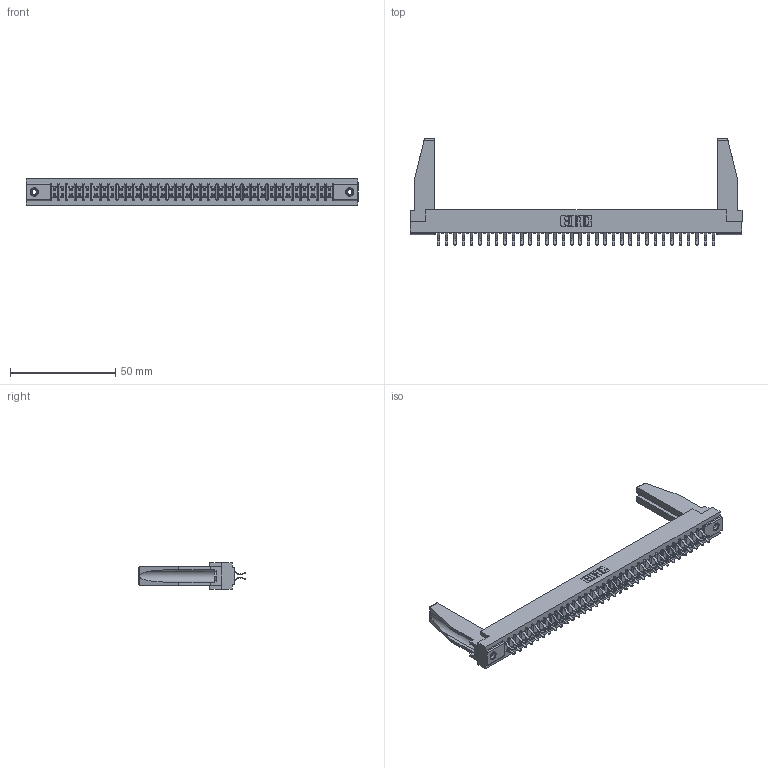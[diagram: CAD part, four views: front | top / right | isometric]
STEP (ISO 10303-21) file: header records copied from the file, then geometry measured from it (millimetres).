
FILE_DESCRIPTION (( 'STEP AP203' ), '1' );
FILE_NAME ('357-068-456-278.STEP', '2020-10-04T23:27:22', ( '' ), ( '' ), 'SwSTEP 2.0', 'SolidWorks 2020', '' );
FILE_SCHEMA (( 'CONFIG_CONTROL_DESIGN' ));
Length unit declared in the file: inch
Products named in the file (5): 307-220-078; 307 Part_.156 Dia Mounting Holes; 307-290-001_556; 345-250-001_345-250-001-102; 357-068-456-278
Assembly tree (73 placements, depth 2):
  357-068-456-278
    307 Part_.156 Dia Mounting Holes
    307-290-001_556  x68
    307-220-078  x2
    345-250-001_345-250-001-102  x2
Bounding box: 157.73 x 50.67 x 12.7 mm (x, y, z)
Volume: 20697.5 mm3; surface area: 23924.4 mm2
Topology: 73 solids, 73 shells, 3683 faces, 10309 edges, 6678 vertices
Faces by surface type: plane 2398, cylinder 1199, sphere 70, cone 12, torus 4
Entity records: 33765 total; most frequent: CARTESIAN_POINT 5536, ORIENTED_EDGE 5444, DIRECTION 5380, EDGE_CURVE 2722, LINE 2088, VECTOR 2088, VERTEX_POINT 1760, AXIS2_PLACEMENT_3D 1646
